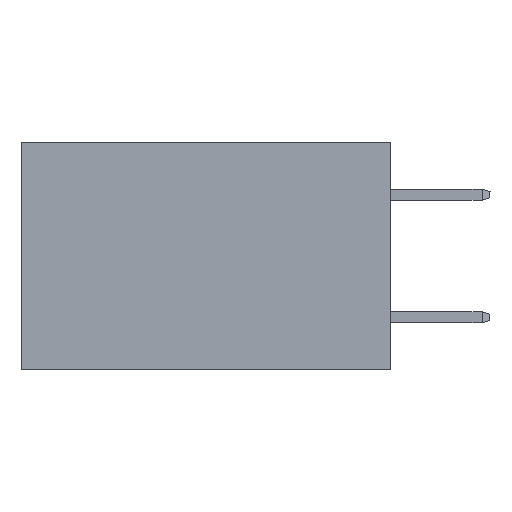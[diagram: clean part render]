
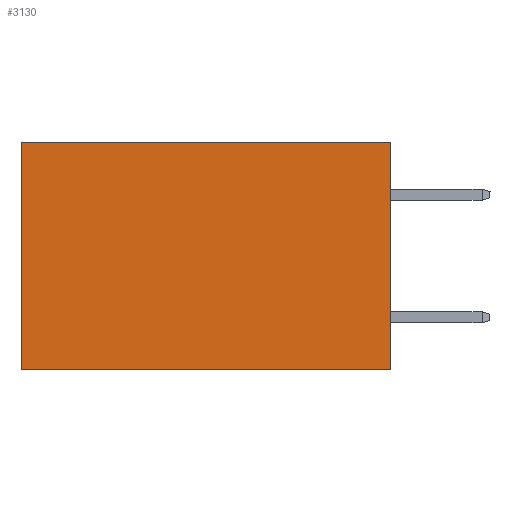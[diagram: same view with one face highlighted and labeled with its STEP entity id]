
A CAD part, left-side view. The second image highlights one B-rep face of the part: STEP entity #3130.
In plain terms, the highlighted planar face has unit normal (-1, 0, 0).
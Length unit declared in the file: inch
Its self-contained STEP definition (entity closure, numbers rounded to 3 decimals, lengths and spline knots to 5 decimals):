
#1131 = DIRECTION ( 'NONE',  ( 1., 0., 0. ) ) ;
#1535 = VERTEX_POINT ( 'NONE', #10013 ) ;
#1617 = VECTOR ( 'NONE', #10761, 39.37008 ) ;
#1850 = CARTESIAN_POINT ( 'NONE',  ( 0.2875, 0., -0.37 ) ) ;
#2478 = EDGE_CURVE ( 'NONE', #4385, #12365, #7993, .T. ) ;
#3130 = ADVANCED_FACE ( 'NONE', ( #16168 ), #15139, .F. ) ;
#3355 = ORIENTED_EDGE ( 'NONE', *, *, #2478, .T. ) ;
#4358 = VECTOR ( 'NONE', #8209, 39.37008 ) ;
#4385 = VERTEX_POINT ( 'NONE', #12628 ) ;
#4499 = DIRECTION ( 'NONE',  ( 0., 0., -1. ) ) ;
#5412 = CARTESIAN_POINT ( 'NONE',  ( 0.2875, 0., 0. ) ) ;
#6063 = ORIENTED_EDGE ( 'NONE', *, *, #10861, .F. ) ;
#6545 = ORIENTED_EDGE ( 'NONE', *, *, #15982, .F. ) ;
#6848 = VERTEX_POINT ( 'NONE', #14545 ) ;
#7069 = CARTESIAN_POINT ( 'NONE',  ( 0.2875, 0., 0. ) ) ;
#7384 = ORIENTED_EDGE ( 'NONE', *, *, #16004, .T. ) ;
#7965 = EDGE_LOOP ( 'NONE', ( #7384, #6063, #6545, #3355 ) ) ;
#7993 = LINE ( 'NONE', #7069, #1617 ) ;
#8187 = CARTESIAN_POINT ( 'NONE',  ( 0.2875, 0.6, 0. ) ) ;
#8209 = DIRECTION ( 'NONE',  ( 0., 1., 0. ) ) ;
#9578 = VECTOR ( 'NONE', #4499, 39.37008 ) ;
#10013 = CARTESIAN_POINT ( 'NONE',  ( 0.2875, 0., -0.37 ) ) ;
#10761 = DIRECTION ( 'NONE',  ( 0., 1., 0. ) ) ;
#10861 = EDGE_CURVE ( 'NONE', #1535, #6848, #11758, .T. ) ;
#11731 = CARTESIAN_POINT ( 'NONE',  ( 0.2875, 0.6, 0. ) ) ;
#11758 = LINE ( 'NONE', #1850, #4358 ) ;
#12365 = VERTEX_POINT ( 'NONE', #11731 ) ;
#12628 = CARTESIAN_POINT ( 'NONE',  ( 0.2875, 0., 0. ) ) ;
#12963 = LINE ( 'NONE', #8187, #15553 ) ;
#13245 = AXIS2_PLACEMENT_3D ( 'NONE', #16406, #1131, #13900 ) ;
#13900 = DIRECTION ( 'NONE',  ( 0., 0., -1. ) ) ;
#14545 = CARTESIAN_POINT ( 'NONE',  ( 0.2875, 0.6, -0.37 ) ) ;
#15139 = PLANE ( 'NONE',  #13245 ) ;
#15553 = VECTOR ( 'NONE', #15993, 39.37008 ) ;
#15982 = EDGE_CURVE ( 'NONE', #4385, #1535, #16346, .T. ) ;
#15993 = DIRECTION ( 'NONE',  ( 0., 0., -1. ) ) ;
#16004 = EDGE_CURVE ( 'NONE', #12365, #6848, #12963, .T. ) ;
#16168 = FACE_OUTER_BOUND ( 'NONE', #7965, .T. ) ;
#16346 = LINE ( 'NONE', #5412, #9578 ) ;
#16406 = CARTESIAN_POINT ( 'NONE',  ( 0.2875, 0., 0. ) ) ;
